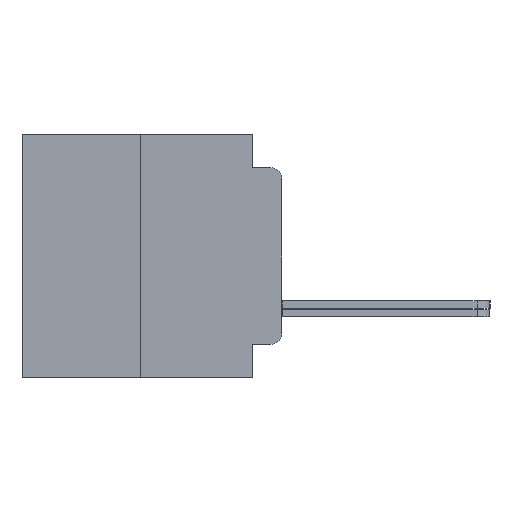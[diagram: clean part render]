
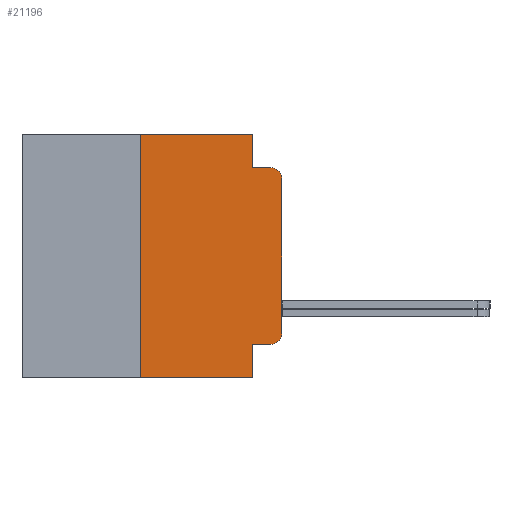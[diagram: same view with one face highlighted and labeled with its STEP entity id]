
A CAD part, left-side view. The second image highlights one B-rep face of the part: STEP entity #21196.
In plain terms, the highlighted planar face has unit normal (-1, 0, 0).
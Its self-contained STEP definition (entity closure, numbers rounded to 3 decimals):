
#66 = AXIS2_PLACEMENT_3D ( 'NONE', #7802, #25109, #9942 ) ;
#681 = EDGE_CURVE ( 'NONE', #9298, #2573, #14773, .T. ) ;
#919 = CARTESIAN_POINT ( 'NONE',  ( -75.603, 1.295, 0. ) ) ;
#937 = DIRECTION ( 'NONE',  ( 0., -1., 0. ) ) ;
#1851 = LINE ( 'NONE', #9269, #9522 ) ;
#2477 = ORIENTED_EDGE ( 'NONE', *, *, #7117, .T. ) ;
#2486 = LINE ( 'NONE', #919, #11128 ) ;
#2573 = VERTEX_POINT ( 'NONE', #4455 ) ;
#2628 = ORIENTED_EDGE ( 'NONE', *, *, #26884, .F. ) ;
#4050 = EDGE_CURVE ( 'NONE', #9298, #8109, #14762, .T. ) ;
#4455 = CARTESIAN_POINT ( 'NONE',  ( -75.603, 6.35, 5.486 ) ) ;
#5053 = DIRECTION ( 'NONE',  ( 0., 0., -1. ) ) ;
#5369 = CARTESIAN_POINT ( 'NONE',  ( -75.603, 0., -3.467 ) ) ;
#5437 = LINE ( 'NONE', #24292, #12084 ) ;
#6265 = CARTESIAN_POINT ( 'NONE',  ( -75.603, 0., 5.486 ) ) ;
#6426 = CARTESIAN_POINT ( 'NONE',  ( -75.603, 1.295, -5.486 ) ) ;
#6489 = VERTEX_POINT ( 'NONE', #5369 ) ;
#6788 = VERTEX_POINT ( 'NONE', #10662 ) ;
#7117 = EDGE_CURVE ( 'NONE', #20334, #26411, #20545, .T. ) ;
#7802 = CARTESIAN_POINT ( 'NONE',  ( -75.603, 0.508, 3.467 ) ) ;
#7881 = EDGE_CURVE ( 'NONE', #22393, #12929, #1851, .T. ) ;
#8013 = DIRECTION ( 'NONE',  ( 0., 0., 1. ) ) ;
#8109 = VERTEX_POINT ( 'NONE', #6426 ) ;
#8311 = VERTEX_POINT ( 'NONE', #18113 ) ;
#8474 = DIRECTION ( 'NONE',  ( 1., 0., 0. ) ) ;
#8504 = EDGE_LOOP ( 'NONE', ( #2477, #24108, #26482, #22108, #21100, #24709, #2628, #11109, #23028, #8603 ) ) ;
#8510 = DIRECTION ( 'NONE',  ( 0., 0., -1. ) ) ;
#8603 = ORIENTED_EDGE ( 'NONE', *, *, #9165, .F. ) ;
#8732 = VECTOR ( 'NONE', #937, 1000. ) ;
#9165 = EDGE_CURVE ( 'NONE', #20334, #8109, #2486, .T. ) ;
#9269 = CARTESIAN_POINT ( 'NONE',  ( -75.603, 1.295, 0. ) ) ;
#9298 = VERTEX_POINT ( 'NONE', #17757 ) ;
#9522 = VECTOR ( 'NONE', #5053, 1000. ) ;
#9537 = CARTESIAN_POINT ( 'NONE',  ( -75.603, 11.684, -5.486 ) ) ;
#9942 = DIRECTION ( 'NONE',  ( 0., 0., -1. ) ) ;
#10630 = DIRECTION ( 'NONE',  ( -1., 0., 0. ) ) ;
#10662 = CARTESIAN_POINT ( 'NONE',  ( -75.603, 0., 3.467 ) ) ;
#10986 = CIRCLE ( 'NONE', #15901, 0.508 ) ;
#11109 = ORIENTED_EDGE ( 'NONE', *, *, #681, .F. ) ;
#11128 = VECTOR ( 'NONE', #21439, 1000. ) ;
#11893 = VECTOR ( 'NONE', #23069, 1000. ) ;
#12084 = VECTOR ( 'NONE', #26470, 1000. ) ;
#12297 = CARTESIAN_POINT ( 'NONE',  ( -75.603, 6.35, -5.486 ) ) ;
#12744 = PLANE ( 'NONE',  #16644 ) ;
#12929 = VERTEX_POINT ( 'NONE', #27430 ) ;
#13729 = VECTOR ( 'NONE', #22091, 1000. ) ;
#14425 = CARTESIAN_POINT ( 'NONE',  ( -75.603, 1.295, -3.975 ) ) ;
#14568 = EDGE_CURVE ( 'NONE', #12929, #8311, #27355, .T. ) ;
#14762 = LINE ( 'NONE', #9537, #13729 ) ;
#14773 = LINE ( 'NONE', #12297, #16406 ) ;
#15104 = CARTESIAN_POINT ( 'NONE',  ( -75.603, 0.508, -3.467 ) ) ;
#15901 = AXIS2_PLACEMENT_3D ( 'NONE', #15104, #10630, #8510 ) ;
#16406 = VECTOR ( 'NONE', #8013, 1000. ) ;
#16644 = AXIS2_PLACEMENT_3D ( 'NONE', #18780, #8474, #20938 ) ;
#16719 = CARTESIAN_POINT ( 'NONE',  ( -75.603, 0.508, -3.975 ) ) ;
#17012 = DIRECTION ( 'NONE',  ( 0., 0., 1. ) ) ;
#17297 = CIRCLE ( 'NONE', #66, 0.508 ) ;
#17435 = LINE ( 'NONE', #6265, #24457 ) ;
#17757 = CARTESIAN_POINT ( 'NONE',  ( -75.603, 6.35, -5.486 ) ) ;
#18113 = CARTESIAN_POINT ( 'NONE',  ( -75.603, 0.508, 3.975 ) ) ;
#18780 = CARTESIAN_POINT ( 'NONE',  ( -75.603, 11.684, 5.486 ) ) ;
#19572 = EDGE_CURVE ( 'NONE', #6489, #6788, #17435, .T. ) ;
#20334 = VERTEX_POINT ( 'NONE', #21300 ) ;
#20545 = LINE ( 'NONE', #14425, #11893 ) ;
#20889 = CARTESIAN_POINT ( 'NONE',  ( -75.603, 1.295, 5.486 ) ) ;
#20938 = DIRECTION ( 'NONE',  ( 0., 0., -1. ) ) ;
#21100 = ORIENTED_EDGE ( 'NONE', *, *, #14568, .F. ) ;
#21196 = ADVANCED_FACE ( 'NONE', ( #22362 ), #12744, .F. ) ;
#21300 = CARTESIAN_POINT ( 'NONE',  ( -75.603, 1.295, -3.975 ) ) ;
#21439 = DIRECTION ( 'NONE',  ( 0., 0., -1. ) ) ;
#21671 = EDGE_CURVE ( 'NONE', #6788, #8311, #17297, .T. ) ;
#22091 = DIRECTION ( 'NONE',  ( 0., -1., 0. ) ) ;
#22108 = ORIENTED_EDGE ( 'NONE', *, *, #21671, .T. ) ;
#22362 = FACE_OUTER_BOUND ( 'NONE', #8504, .T. ) ;
#22393 = VERTEX_POINT ( 'NONE', #20889 ) ;
#23028 = ORIENTED_EDGE ( 'NONE', *, *, #4050, .T. ) ;
#23069 = DIRECTION ( 'NONE',  ( 0., -1., 0. ) ) ;
#23492 = EDGE_CURVE ( 'NONE', #26411, #6489, #10986, .T. ) ;
#24087 = CARTESIAN_POINT ( 'NONE',  ( -75.603, 1.295, 3.975 ) ) ;
#24108 = ORIENTED_EDGE ( 'NONE', *, *, #23492, .T. ) ;
#24292 = CARTESIAN_POINT ( 'NONE',  ( -75.603, 11.684, 5.486 ) ) ;
#24457 = VECTOR ( 'NONE', #17012, 1000. ) ;
#24709 = ORIENTED_EDGE ( 'NONE', *, *, #7881, .F. ) ;
#25109 = DIRECTION ( 'NONE',  ( -1., 0., 0. ) ) ;
#26411 = VERTEX_POINT ( 'NONE', #16719 ) ;
#26470 = DIRECTION ( 'NONE',  ( 0., -1., 0. ) ) ;
#26482 = ORIENTED_EDGE ( 'NONE', *, *, #19572, .T. ) ;
#26884 = EDGE_CURVE ( 'NONE', #2573, #22393, #5437, .T. ) ;
#27355 = LINE ( 'NONE', #24087, #8732 ) ;
#27430 = CARTESIAN_POINT ( 'NONE',  ( -75.603, 1.295, 3.975 ) ) ;
